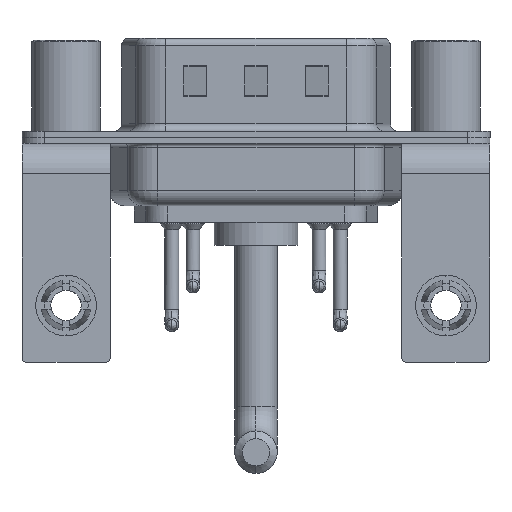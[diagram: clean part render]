
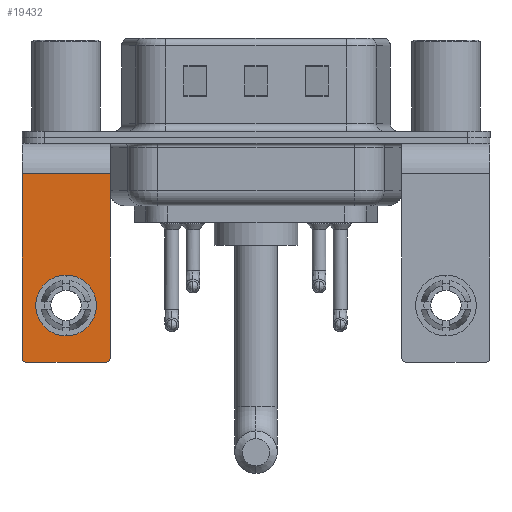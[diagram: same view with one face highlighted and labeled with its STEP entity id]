
A CAD part, front view. The second image highlights one B-rep face of the part: STEP entity #19432.
In plain terms, the highlighted planar face has unit normal (0, -1, 0).
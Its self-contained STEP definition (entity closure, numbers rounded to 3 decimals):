
#130 = DIRECTION ( 'NONE',  ( 0., 0., 1. ) ) ;
#309 = CARTESIAN_POINT ( 'NONE',  ( 2.9, -6.25, -2.4 ) ) ;
#474 = EDGE_CURVE ( 'NONE', #5775, #7956, #7954, .T. ) ;
#726 = EDGE_LOOP ( 'NONE', ( #4346, #20606 ) ) ;
#1082 = AXIS2_PLACEMENT_3D ( 'NONE', #1325, #8527, #13468 ) ;
#1325 = CARTESIAN_POINT ( 'NONE',  ( 2.65, -6.25, -14.55 ) ) ;
#1540 = FACE_BOUND ( 'NONE', #726, .T. ) ;
#1867 = CARTESIAN_POINT ( 'NONE',  ( -2.65, -6.25, -14.55 ) ) ;
#3207 = CARTESIAN_POINT ( 'NONE',  ( 2.9, -6.25, -2.4 ) ) ;
#3804 = LINE ( 'NONE', #10862, #10562 ) ;
#4346 = ORIENTED_EDGE ( 'NONE', *, *, #21618, .T. ) ;
#4363 = VERTEX_POINT ( 'NONE', #10178 ) ;
#4387 = LINE ( 'NONE', #6114, #12452 ) ;
#5160 = EDGE_CURVE ( 'NONE', #7654, #17450, #7408, .T. ) ;
#5196 = DIRECTION ( 'NONE',  ( 0., 0., 1. ) ) ;
#5511 = ORIENTED_EDGE ( 'NONE', *, *, #22789, .T. ) ;
#5701 = ORIENTED_EDGE ( 'NONE', *, *, #5160, .T. ) ;
#5775 = VERTEX_POINT ( 'NONE', #15875 ) ;
#6114 = CARTESIAN_POINT ( 'NONE',  ( 2.9, -6.25, -14.8 ) ) ;
#6186 = AXIS2_PLACEMENT_3D ( 'NONE', #22636, #15930, #5196 ) ;
#6488 = VECTOR ( 'NONE', #7397, 1000. ) ;
#7294 = CIRCLE ( 'NONE', #6186, 2. ) ;
#7397 = DIRECTION ( 'NONE',  ( 0., 0., -1. ) ) ;
#7408 = CIRCLE ( 'NONE', #1082, 0.25 ) ;
#7654 = VERTEX_POINT ( 'NONE', #12462 ) ;
#7954 = CIRCLE ( 'NONE', #14941, 2. ) ;
#7956 = VERTEX_POINT ( 'NONE', #19129 ) ;
#8243 = DIRECTION ( 'NONE',  ( 0., 0., 1. ) ) ;
#8527 = DIRECTION ( 'NONE',  ( 0., -1., 0. ) ) ;
#8626 = FACE_OUTER_BOUND ( 'NONE', #18090, .T. ) ;
#8690 = EDGE_CURVE ( 'NONE', #7654, #4363, #4387, .T. ) ;
#8862 = PLANE ( 'NONE',  #14219 ) ;
#8951 = DIRECTION ( 'NONE',  ( 0., 0., 1. ) ) ;
#9056 = CARTESIAN_POINT ( 'NONE',  ( 2.9, -6.25, -2.4 ) ) ;
#9156 = ORIENTED_EDGE ( 'NONE', *, *, #11258, .F. ) ;
#9756 = DIRECTION ( 'NONE',  ( 0., 1., 0. ) ) ;
#10096 = CARTESIAN_POINT ( 'NONE',  ( 0., -6.25, -11.07 ) ) ;
#10178 = CARTESIAN_POINT ( 'NONE',  ( -2.65, -6.25, -14.8 ) ) ;
#10562 = VECTOR ( 'NONE', #16172, 1000. ) ;
#10596 = VECTOR ( 'NONE', #10780, 1000. ) ;
#10725 = VERTEX_POINT ( 'NONE', #3207 ) ;
#10780 = DIRECTION ( 'NONE',  ( -1., 0., 0. ) ) ;
#10862 = CARTESIAN_POINT ( 'NONE',  ( -2.9, -6.25, -2.4 ) ) ;
#11089 = CARTESIAN_POINT ( 'NONE',  ( -2.9, -6.25, -2.4 ) ) ;
#11258 = EDGE_CURVE ( 'NONE', #10725, #17450, #12695, .T. ) ;
#12452 = VECTOR ( 'NONE', #18584, 1000. ) ;
#12462 = CARTESIAN_POINT ( 'NONE',  ( 2.65, -6.25, -14.8 ) ) ;
#12523 = EDGE_CURVE ( 'NONE', #10725, #18755, #17720, .T. ) ;
#12637 = DIRECTION ( 'NONE',  ( 0., 1., 0. ) ) ;
#12695 = LINE ( 'NONE', #309, #6488 ) ;
#13468 = DIRECTION ( 'NONE',  ( 0., 0., 1. ) ) ;
#14219 = AXIS2_PLACEMENT_3D ( 'NONE', #15891, #12637, #130 ) ;
#14635 = CARTESIAN_POINT ( 'NONE',  ( -2.9, -6.25, -14.55 ) ) ;
#14941 = AXIS2_PLACEMENT_3D ( 'NONE', #10096, #9756, #8243 ) ;
#15864 = ORIENTED_EDGE ( 'NONE', *, *, #8690, .F. ) ;
#15875 = CARTESIAN_POINT ( 'NONE',  ( 0., -6.25, -9.07 ) ) ;
#15891 = CARTESIAN_POINT ( 'NONE',  ( 2.9, -6.25, -2.4 ) ) ;
#15930 = DIRECTION ( 'NONE',  ( 0., 1., 0. ) ) ;
#16172 = DIRECTION ( 'NONE',  ( 0., 0., -1. ) ) ;
#16181 = CIRCLE ( 'NONE', #19496, 0.25 ) ;
#17450 = VERTEX_POINT ( 'NONE', #21702 ) ;
#17720 = LINE ( 'NONE', #9056, #10596 ) ;
#17824 = DIRECTION ( 'NONE',  ( 0., -1., 0. ) ) ;
#18090 = EDGE_LOOP ( 'NONE', ( #20306, #5511, #15864, #5701, #9156, #19319 ) ) ;
#18584 = DIRECTION ( 'NONE',  ( -1., 0., 0. ) ) ;
#18745 = EDGE_CURVE ( 'NONE', #18755, #20468, #3804, .T. ) ;
#18755 = VERTEX_POINT ( 'NONE', #11089 ) ;
#19129 = CARTESIAN_POINT ( 'NONE',  ( 0., -6.25, -13.07 ) ) ;
#19319 = ORIENTED_EDGE ( 'NONE', *, *, #12523, .T. ) ;
#19432 = ADVANCED_FACE ( 'NONE', ( #1540, #8626 ), #8862, .F. ) ;
#19496 = AXIS2_PLACEMENT_3D ( 'NONE', #1867, #17824, #8951 ) ;
#20306 = ORIENTED_EDGE ( 'NONE', *, *, #18745, .T. ) ;
#20468 = VERTEX_POINT ( 'NONE', #14635 ) ;
#20606 = ORIENTED_EDGE ( 'NONE', *, *, #474, .T. ) ;
#21618 = EDGE_CURVE ( 'NONE', #7956, #5775, #7294, .T. ) ;
#21702 = CARTESIAN_POINT ( 'NONE',  ( 2.9, -6.25, -14.55 ) ) ;
#22636 = CARTESIAN_POINT ( 'NONE',  ( 0., -6.25, -11.07 ) ) ;
#22789 = EDGE_CURVE ( 'NONE', #20468, #4363, #16181, .T. ) ;
